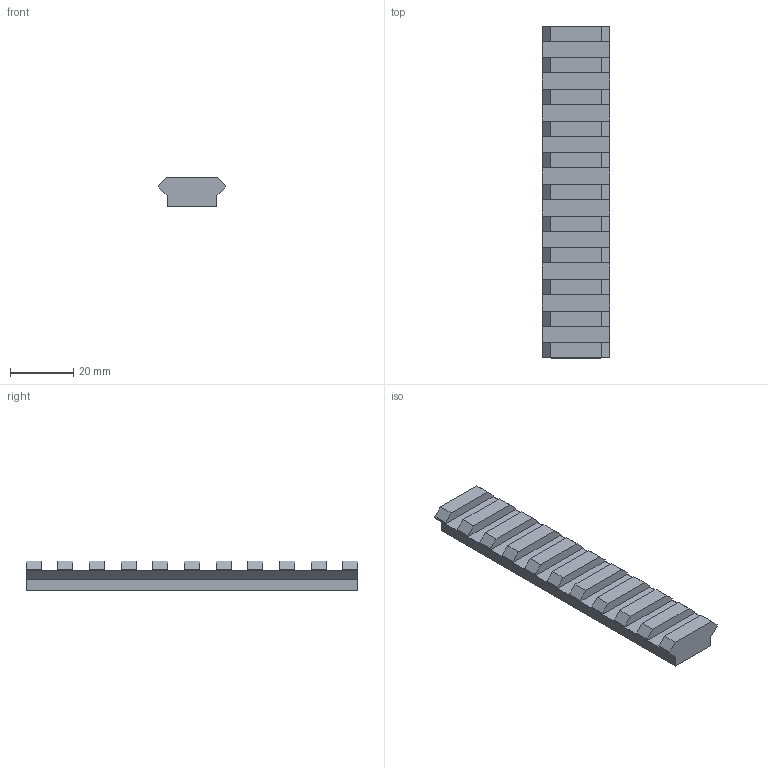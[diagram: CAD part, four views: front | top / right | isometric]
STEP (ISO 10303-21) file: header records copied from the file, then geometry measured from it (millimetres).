
FILE_DESCRIPTION(/* description */ (''),/* implementation_level */ '2;1');
FILE_NAME(/* name */ '10 Slot Picatinny Rail.step',/* time_stamp */ '2021-04-28T07:41:51-04:00',/* author */ (''),/* organization */ (''),/* preprocessor_version */ 'ST-DEVELOPER v18.1',/* originating_system */ 'Autodesk Translation Framework v10.6.0.1341',/* authorisation */ '');
FILE_SCHEMA (('AUTOMOTIVE_DESIGN { 1 0 10303 214 3 1 1 }'));
Length unit declared in the file: millimetre
Products named in the file (1): 10 Slot Picatinny Rail
Bounding box: 21.21 x 104.75 x 9.32 mm (x, y, z)
Volume: 14206.1 mm3; surface area: 7060.4 mm2
Topology: 1 solids, 1 shells, 72 faces, 210 edges, 140 vertices
Faces by surface type: plane 72
Entity records: 2374 total; most frequent: CARTESIAN_POINT 423, ORIENTED_EDGE 420, DIRECTION 356, LINE 210, VECTOR 210, EDGE_CURVE 210, VERTEX_POINT 140, AXIS2_PLACEMENT_3D 73
